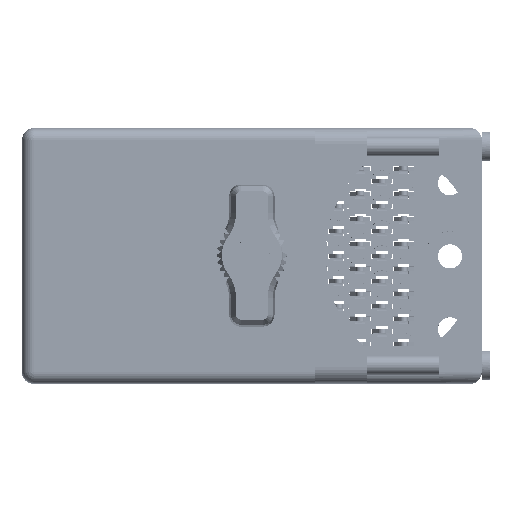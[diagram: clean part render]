
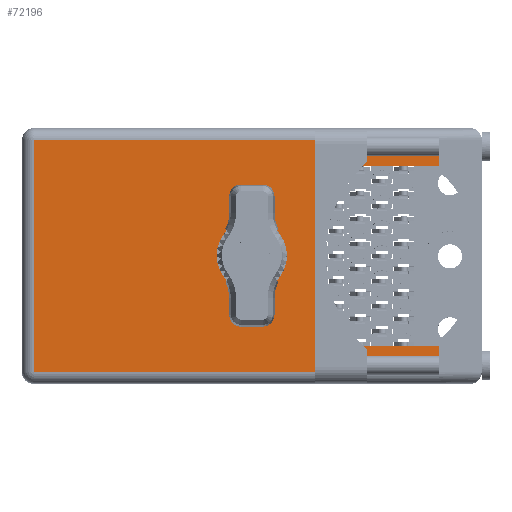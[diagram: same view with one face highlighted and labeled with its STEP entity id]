
A CAD part, top view. The second image highlights one B-rep face of the part: STEP entity #72196.
In plain terms, the highlighted face is planar.
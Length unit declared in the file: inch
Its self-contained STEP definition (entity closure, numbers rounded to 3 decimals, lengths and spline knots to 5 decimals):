
#4367 = LINE ( 'NONE', #22355, #102564 ) ;
#5359 = VECTOR ( 'NONE', #68029, 39.37008 ) ;
#5760 = CARTESIAN_POINT ( 'NONE',  ( 0.4075, 1.93, 0.54 ) ) ;
#5880 = EDGE_LOOP ( 'NONE', ( #92388, #61643 ) ) ;
#7380 = CARTESIAN_POINT ( 'NONE',  ( 1.1215, 1.93, -0.54 ) ) ;
#9800 = VERTEX_POINT ( 'NONE', #99082 ) ;
#13808 = EDGE_CURVE ( 'NONE', #57819, #50084, #29609, .T. ) ;
#15919 = CARTESIAN_POINT ( 'NONE',  ( 1.1215, 1.93, -0.54 ) ) ;
#16433 = VERTEX_POINT ( 'NONE', #67202 ) ;
#17020 = DIRECTION ( 'NONE',  ( 0., 0., 1. ) ) ;
#17910 = EDGE_CURVE ( 'NONE', #89376, #102836, #56900, .T. ) ;
#20026 = DIRECTION ( 'NONE',  ( 0., 0., -1. ) ) ;
#22355 = CARTESIAN_POINT ( 'NONE',  ( 1.1215, 1.93, -0.765 ) ) ;
#25703 = EDGE_CURVE ( 'NONE', #16433, #57826, #44911, .T. ) ;
#28871 = CARTESIAN_POINT ( 'NONE',  ( 0.4075, 1.93, -0.54 ) ) ;
#29390 = EDGE_CURVE ( 'NONE', #65438, #81860, #37110, .T. ) ;
#29395 = EDGE_LOOP ( 'NONE', ( #95096, #87093, #74503, #80316, #85135, #54199, #43645, #46190 ) ) ;
#29609 = LINE ( 'NONE', #45923, #62751 ) ;
#33665 = LINE ( 'NONE', #28871, #61854 ) ;
#35519 = PLANE ( 'NONE',  #85445 ) ;
#36609 = DIRECTION ( 'NONE',  ( -1., 0., 0. ) ) ;
#37110 = CIRCLE ( 'NONE', #61898, 0.17 ) ;
#37764 = EDGE_CURVE ( 'NONE', #16433, #102836, #80444, .T. ) ;
#39407 = CARTESIAN_POINT ( 'NONE',  ( 0.4075, 1.93, -0.54 ) ) ;
#41934 = DIRECTION ( 'NONE',  ( 0., 1., 0. ) ) ;
#42354 = CARTESIAN_POINT ( 'NONE',  ( -1.3775, 1.93, -0.695 ) ) ;
#42636 = DIRECTION ( 'NONE',  ( 0., 1., 0. ) ) ;
#43645 = ORIENTED_EDGE ( 'NONE', *, *, #37764, .F. ) ;
#44382 = CARTESIAN_POINT ( 'NONE',  ( 0., 1.93, -0.17 ) ) ;
#44911 = LINE ( 'NONE', #42354, #5359 ) ;
#45923 = CARTESIAN_POINT ( 'NONE',  ( 1.1215, 1.93, 0.54 ) ) ;
#46190 = ORIENTED_EDGE ( 'NONE', *, *, #25703, .T. ) ;
#46995 = FACE_OUTER_BOUND ( 'NONE', #29395, .T. ) ;
#47203 = DIRECTION ( 'NONE',  ( 0., 0., 1. ) ) ;
#48131 = EDGE_CURVE ( 'NONE', #57826, #9800, #67101, .T. ) ;
#50084 = VERTEX_POINT ( 'NONE', #5760 ) ;
#50472 = CARTESIAN_POINT ( 'NONE',  ( 0., 1.93, 0. ) ) ;
#52115 = FACE_BOUND ( 'NONE', #5880, .T. ) ;
#53772 = DIRECTION ( 'NONE',  ( -1., 0., 0. ) ) ;
#54199 = ORIENTED_EDGE ( 'NONE', *, *, #17910, .T. ) ;
#56129 = EDGE_CURVE ( 'NONE', #57819, #84717, #4367, .T. ) ;
#56900 = LINE ( 'NONE', #7380, #92628 ) ;
#57819 = VERTEX_POINT ( 'NONE', #75470 ) ;
#57826 = VERTEX_POINT ( 'NONE', #59484 ) ;
#58780 = VECTOR ( 'NONE', #17020, 39.37008 ) ;
#59204 = EDGE_CURVE ( 'NONE', #9800, #84717, #105492, .T. ) ;
#59484 = CARTESIAN_POINT ( 'NONE',  ( -1.3075, 1.93, -0.695 ) ) ;
#61643 = ORIENTED_EDGE ( 'NONE', *, *, #29390, .F. ) ;
#61854 = VECTOR ( 'NONE', #20026, 39.37008 ) ;
#61898 = AXIS2_PLACEMENT_3D ( 'NONE', #50472, #42636, #99679 ) ;
#62145 = VECTOR ( 'NONE', #77764, 39.37008 ) ;
#62751 = VECTOR ( 'NONE', #53772, 39.37008 ) ;
#64306 = CARTESIAN_POINT ( 'NONE',  ( -1.3075, 1.93, -0.765 ) ) ;
#65438 = VERTEX_POINT ( 'NONE', #44382 ) ;
#67101 = LINE ( 'NONE', #64306, #69678 ) ;
#67202 = CARTESIAN_POINT ( 'NONE',  ( 1.1215, 1.93, -0.695 ) ) ;
#68029 = DIRECTION ( 'NONE',  ( -1., 0., 0. ) ) ;
#68300 = DIRECTION ( 'NONE',  ( 0., 1., 0. ) ) ;
#68803 = EDGE_CURVE ( 'NONE', #81860, #65438, #105367, .T. ) ;
#69678 = VECTOR ( 'NONE', #47203, 39.37008 ) ;
#71340 = CARTESIAN_POINT ( 'NONE',  ( 1.1215, 1.93, 0.695 ) ) ;
#72196 = ADVANCED_FACE ( 'NONE', ( #46995, #52115 ), #35519, .T. ) ;
#74503 = ORIENTED_EDGE ( 'NONE', *, *, #56129, .F. ) ;
#75470 = CARTESIAN_POINT ( 'NONE',  ( 1.1215, 1.93, 0.54 ) ) ;
#77764 = DIRECTION ( 'NONE',  ( 1., 0., 0. ) ) ;
#78125 = CARTESIAN_POINT ( 'NONE',  ( 1.1215, 1.93, 0.695 ) ) ;
#80316 = ORIENTED_EDGE ( 'NONE', *, *, #13808, .T. ) ;
#80444 = LINE ( 'NONE', #81473, #58780 ) ;
#81473 = CARTESIAN_POINT ( 'NONE',  ( 1.1215, 1.93, -0.765 ) ) ;
#81860 = VERTEX_POINT ( 'NONE', #105582 ) ;
#82567 = CARTESIAN_POINT ( 'NONE',  ( 0., 1.93, 0. ) ) ;
#83629 = DIRECTION ( 'NONE',  ( 0., 0., 1. ) ) ;
#84717 = VERTEX_POINT ( 'NONE', #71340 ) ;
#85135 = ORIENTED_EDGE ( 'NONE', *, *, #85386, .T. ) ;
#85386 = EDGE_CURVE ( 'NONE', #50084, #89376, #33665, .T. ) ;
#85445 = AXIS2_PLACEMENT_3D ( 'NONE', #92551, #68300, #36609 ) ;
#86894 = DIRECTION ( 'NONE',  ( 1., 0., 0. ) ) ;
#87093 = ORIENTED_EDGE ( 'NONE', *, *, #59204, .T. ) ;
#89376 = VERTEX_POINT ( 'NONE', #39407 ) ;
#92013 = AXIS2_PLACEMENT_3D ( 'NONE', #82567, #41934, #83629 ) ;
#92388 = ORIENTED_EDGE ( 'NONE', *, *, #68803, .F. ) ;
#92551 = CARTESIAN_POINT ( 'NONE',  ( -1.3775, 1.93, -0.765 ) ) ;
#92628 = VECTOR ( 'NONE', #86894, 39.37008 ) ;
#95096 = ORIENTED_EDGE ( 'NONE', *, *, #48131, .T. ) ;
#99082 = CARTESIAN_POINT ( 'NONE',  ( -1.3075, 1.93, 0.695 ) ) ;
#99679 = DIRECTION ( 'NONE',  ( 0., 0., 1. ) ) ;
#102564 = VECTOR ( 'NONE', #102926, 39.37008 ) ;
#102836 = VERTEX_POINT ( 'NONE', #15919 ) ;
#102926 = DIRECTION ( 'NONE',  ( 0., 0., 1. ) ) ;
#105367 = CIRCLE ( 'NONE', #92013, 0.17 ) ;
#105492 = LINE ( 'NONE', #78125, #62145 ) ;
#105582 = CARTESIAN_POINT ( 'NONE',  ( 0., 1.93, 0.17 ) ) ;
